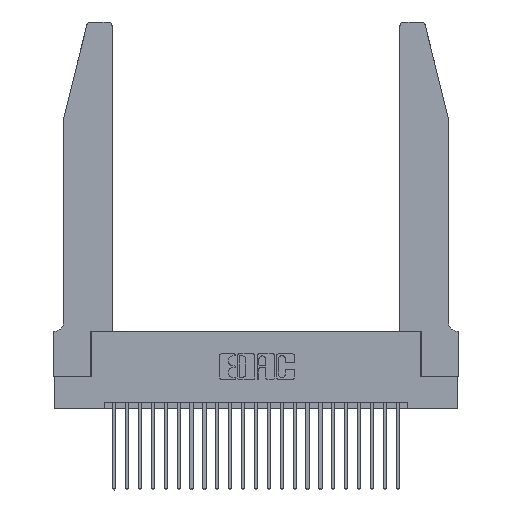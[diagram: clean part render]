
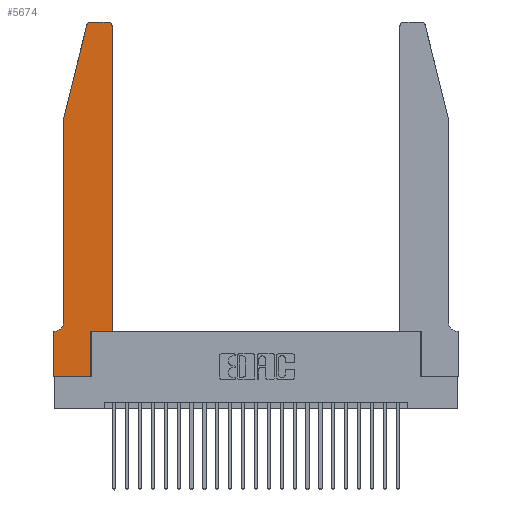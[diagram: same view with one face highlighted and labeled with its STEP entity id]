
A CAD part, top view. The second image highlights one B-rep face of the part: STEP entity #5674.
In plain terms, the highlighted planar face has unit normal (0, 0, 1).
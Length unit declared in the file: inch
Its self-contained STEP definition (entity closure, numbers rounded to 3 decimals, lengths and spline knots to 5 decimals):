
#189 = EDGE_CURVE ( 'NONE', #11948, #20029, #3322, .T. ) ;
#353 = DIRECTION ( 'NONE',  ( 1., 0., 0. ) ) ;
#686 = LINE ( 'NONE', #24895, #21185 ) ;
#1103 = VECTOR ( 'NONE', #353, 39.37008 ) ;
#1137 = CIRCLE ( 'NONE', #13519, 0.03 ) ;
#1378 = ORIENTED_EDGE ( 'NONE', *, *, #189, .T. ) ;
#1415 = ORIENTED_EDGE ( 'NONE', *, *, #13642, .T. ) ;
#2191 = VECTOR ( 'NONE', #17461, 39.37008 ) ;
#3089 = CARTESIAN_POINT ( 'NONE',  ( 0.2865, 0.35, 0.37 ) ) ;
#3322 = LINE ( 'NONE', #8694, #7011 ) ;
#3410 = AXIS2_PLACEMENT_3D ( 'NONE', #13801, #19541, #21395 ) ;
#3504 = CARTESIAN_POINT ( 'NONE',  ( 0.284, 2.72, 0.37 ) ) ;
#3544 = CARTESIAN_POINT ( 'NONE',  ( 0.4505, 0.35, 0.37 ) ) ;
#3639 = ORIENTED_EDGE ( 'NONE', *, *, #5401, .T. ) ;
#4082 = LINE ( 'NONE', #3544, #18226 ) ;
#4206 = VERTEX_POINT ( 'NONE', #13190 ) ;
#4558 = CARTESIAN_POINT ( 'NONE',  ( 0.2865, 0.35, 0.37 ) ) ;
#4679 = LINE ( 'NONE', #16322, #13245 ) ;
#5084 = DIRECTION ( 'NONE',  ( 0., -1., 0. ) ) ;
#5181 = EDGE_CURVE ( 'NONE', #8060, #6366, #13808, .T. ) ;
#5312 = VERTEX_POINT ( 'NONE', #8577 ) ;
#5364 = DIRECTION ( 'NONE',  ( 1., 0., 0. ) ) ;
#5401 = EDGE_CURVE ( 'NONE', #13981, #8060, #23958, .T. ) ;
#5521 = CARTESIAN_POINT ( 'NONE',  ( 0.0755, 2., 0.37 ) ) ;
#5674 = ADVANCED_FACE ( 'NONE', ( #13628 ), #19691, .T. ) ;
#6187 = LINE ( 'NONE', #3089, #21203 ) ;
#6366 = VERTEX_POINT ( 'NONE', #6889 ) ;
#6393 = ORIENTED_EDGE ( 'NONE', *, *, #13784, .T. ) ;
#6668 = EDGE_CURVE ( 'NONE', #16743, #22323, #4082, .T. ) ;
#6889 = CARTESIAN_POINT ( 'NONE',  ( 0., 0.35, 0.37 ) ) ;
#6940 = EDGE_CURVE ( 'NONE', #20029, #13981, #25261, .T. ) ;
#7011 = VECTOR ( 'NONE', #12627, 39.37008 ) ;
#7144 = ORIENTED_EDGE ( 'NONE', *, *, #6940, .T. ) ;
#8004 = VERTEX_POINT ( 'NONE', #4558 ) ;
#8060 = VERTEX_POINT ( 'NONE', #22372 ) ;
#8073 = VECTOR ( 'NONE', #21574, 39.37008 ) ;
#8320 = CARTESIAN_POINT ( 'NONE',  ( 0.4505, 2.72, 0.37 ) ) ;
#8472 = CARTESIAN_POINT ( 'NONE',  ( 0., 0., 0.37 ) ) ;
#8577 = CARTESIAN_POINT ( 'NONE',  ( 0.4205, 2.75, 0.37 ) ) ;
#8694 = CARTESIAN_POINT ( 'NONE',  ( 0.0755, 2., 0.37 ) ) ;
#8799 = CARTESIAN_POINT ( 'NONE',  ( 0.2865, 0., 0.37 ) ) ;
#9914 = ORIENTED_EDGE ( 'NONE', *, *, #5181, .T. ) ;
#11237 = EDGE_LOOP ( 'NONE', ( #12335, #25129, #1378, #7144, #3639, #9914, #18499, #1415, #21194, #17929, #23363, #6393 ) ) ;
#11517 = LINE ( 'NONE', #19543, #1103 ) ;
#11948 = VERTEX_POINT ( 'NONE', #25305 ) ;
#11977 = VECTOR ( 'NONE', #25115, 39.37008 ) ;
#12088 = EDGE_CURVE ( 'NONE', #8004, #16743, #4679, .T. ) ;
#12335 = ORIENTED_EDGE ( 'NONE', *, *, #20764, .T. ) ;
#12627 = DIRECTION ( 'NONE',  ( -0.239, -0.971, 0. ) ) ;
#13114 = CARTESIAN_POINT ( 'NONE',  ( 0.0755, 0.35, 0.37 ) ) ;
#13190 = CARTESIAN_POINT ( 'NONE',  ( 0.284, 2.75, 0.37 ) ) ;
#13234 = EDGE_CURVE ( 'NONE', #4206, #11948, #1137, .T. ) ;
#13245 = VECTOR ( 'NONE', #20479, 39.37008 ) ;
#13408 = CARTESIAN_POINT ( 'NONE',  ( 0.0755, 2., 0.37 ) ) ;
#13429 = CARTESIAN_POINT ( 'NONE',  ( 0.0055, 0.42, 0.37 ) ) ;
#13519 = AXIS2_PLACEMENT_3D ( 'NONE', #3504, #19167, #5364 ) ;
#13628 = FACE_OUTER_BOUND ( 'NONE', #11237, .T. ) ;
#13642 = EDGE_CURVE ( 'NONE', #14723, #14317, #11517, .T. ) ;
#13784 = EDGE_CURVE ( 'NONE', #22323, #5312, #14613, .T. ) ;
#13801 = CARTESIAN_POINT ( 'NONE',  ( 0., 0.35, 0.37 ) ) ;
#13808 = LINE ( 'NONE', #13114, #11977 ) ;
#13981 = VERTEX_POINT ( 'NONE', #14808 ) ;
#14003 = CARTESIAN_POINT ( 'NONE',  ( 0.4205, 2.72, 0.37 ) ) ;
#14235 = DIRECTION ( 'NONE',  ( 0., 0., 1. ) ) ;
#14317 = VERTEX_POINT ( 'NONE', #8799 ) ;
#14613 = CIRCLE ( 'NONE', #17778, 0.03 ) ;
#14723 = VERTEX_POINT ( 'NONE', #8472 ) ;
#14808 = CARTESIAN_POINT ( 'NONE',  ( 0.0755, 0.42, 0.37 ) ) ;
#16322 = CARTESIAN_POINT ( 'NONE',  ( 0.4505, 0.35, 0.37 ) ) ;
#16715 = AXIS2_PLACEMENT_3D ( 'NONE', #13429, #17446, #18022 ) ;
#16743 = VERTEX_POINT ( 'NONE', #18513 ) ;
#17446 = DIRECTION ( 'NONE',  ( 0., 0., -1. ) ) ;
#17461 = DIRECTION ( 'NONE',  ( -1., 0., 0. ) ) ;
#17778 = AXIS2_PLACEMENT_3D ( 'NONE', #14003, #14235, #23224 ) ;
#17825 = LINE ( 'NONE', #25183, #2191 ) ;
#17929 = ORIENTED_EDGE ( 'NONE', *, *, #12088, .T. ) ;
#18022 = DIRECTION ( 'NONE',  ( -1., 0., 0. ) ) ;
#18226 = VECTOR ( 'NONE', #23377, 39.37008 ) ;
#18499 = ORIENTED_EDGE ( 'NONE', *, *, #21335, .T. ) ;
#18513 = CARTESIAN_POINT ( 'NONE',  ( 0.4505, 0.35, 0.37 ) ) ;
#19167 = DIRECTION ( 'NONE',  ( 0., 0., 1. ) ) ;
#19541 = DIRECTION ( 'NONE',  ( 0., 0., 1. ) ) ;
#19543 = CARTESIAN_POINT ( 'NONE',  ( 0., 0., 0.37 ) ) ;
#19691 = PLANE ( 'NONE',  #3410 ) ;
#20029 = VERTEX_POINT ( 'NONE', #13408 ) ;
#20421 = EDGE_CURVE ( 'NONE', #14317, #8004, #6187, .T. ) ;
#20479 = DIRECTION ( 'NONE',  ( 1., 0., 0. ) ) ;
#20764 = EDGE_CURVE ( 'NONE', #5312, #4206, #17825, .T. ) ;
#21185 = VECTOR ( 'NONE', #5084, 39.37008 ) ;
#21194 = ORIENTED_EDGE ( 'NONE', *, *, #20421, .T. ) ;
#21203 = VECTOR ( 'NONE', #22504, 39.37008 ) ;
#21335 = EDGE_CURVE ( 'NONE', #6366, #14723, #686, .T. ) ;
#21395 = DIRECTION ( 'NONE',  ( 1., 0., 0. ) ) ;
#21574 = DIRECTION ( 'NONE',  ( 0., -1., 0. ) ) ;
#22323 = VERTEX_POINT ( 'NONE', #8320 ) ;
#22372 = CARTESIAN_POINT ( 'NONE',  ( 0.0055, 0.35, 0.37 ) ) ;
#22504 = DIRECTION ( 'NONE',  ( 0., 1., 0. ) ) ;
#23224 = DIRECTION ( 'NONE',  ( 1., 0., 0. ) ) ;
#23363 = ORIENTED_EDGE ( 'NONE', *, *, #6668, .T. ) ;
#23377 = DIRECTION ( 'NONE',  ( 0., 1., 0. ) ) ;
#23958 = CIRCLE ( 'NONE', #16715, 0.07 ) ;
#24895 = CARTESIAN_POINT ( 'NONE',  ( 0., 0., 0.37 ) ) ;
#25115 = DIRECTION ( 'NONE',  ( -1., 0., 0. ) ) ;
#25129 = ORIENTED_EDGE ( 'NONE', *, *, #13234, .T. ) ;
#25183 = CARTESIAN_POINT ( 'NONE',  ( 0.2605, 2.75, 0.37 ) ) ;
#25261 = LINE ( 'NONE', #5521, #8073 ) ;
#25305 = CARTESIAN_POINT ( 'NONE',  ( 0.25487, 2.72718, 0.37 ) ) ;
